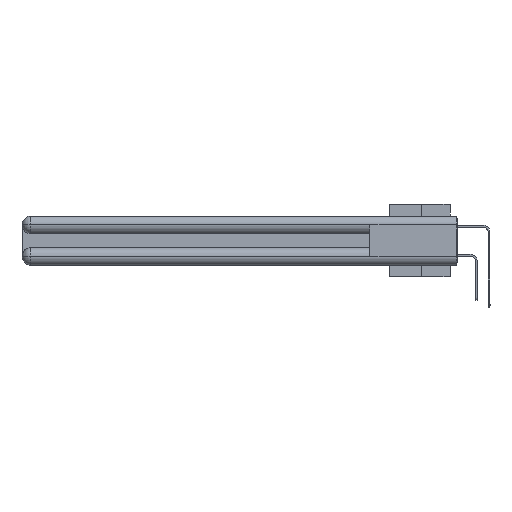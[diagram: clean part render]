
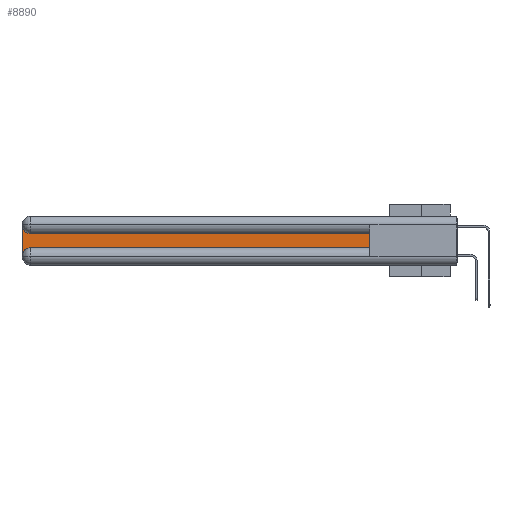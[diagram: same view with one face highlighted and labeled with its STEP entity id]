
A CAD part, left-side view. The second image highlights one B-rep face of the part: STEP entity #8890.
In plain terms, the highlighted planar face has unit normal (-1, 0, 0).
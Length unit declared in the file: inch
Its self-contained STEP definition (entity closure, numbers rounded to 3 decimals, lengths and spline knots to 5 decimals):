
#895 = DIRECTION ( 'NONE',  ( 0., 0., -1. ) ) ;
#2428 = DIRECTION ( 'NONE',  ( 0., 0., -1. ) ) ;
#3851 = CARTESIAN_POINT ( 'NONE',  ( 0.075, 2.94, -0.0625 ) ) ;
#4328 = EDGE_CURVE ( 'NONE', #30875, #16803, #29449, .T. ) ;
#4481 = VECTOR ( 'NONE', #14799, 39.37008 ) ;
#5250 = VERTEX_POINT ( 'NONE', #31226 ) ;
#7126 = DIRECTION ( 'NONE',  ( 1., 0., 0. ) ) ;
#7309 = PLANE ( 'NONE',  #14529 ) ;
#8488 = CARTESIAN_POINT ( 'NONE',  ( 0.075, 3., -0.2175 ) ) ;
#8618 = ORIENTED_EDGE ( 'NONE', *, *, #10377, .T. ) ;
#8878 = EDGE_CURVE ( 'NONE', #16803, #32591, #31275, .T. ) ;
#8890 = ADVANCED_FACE ( 'NONE', ( #12181 ), #7309, .F. ) ;
#8971 = DIRECTION ( 'NONE',  ( 1., 0., 0. ) ) ;
#9100 = CARTESIAN_POINT ( 'NONE',  ( 0.075, 3., -0.2775 ) ) ;
#10290 = CARTESIAN_POINT ( 'NONE',  ( 0.075, 2.94, -0.2175 ) ) ;
#10377 = EDGE_CURVE ( 'NONE', #29912, #5250, #31632, .T. ) ;
#10591 = CARTESIAN_POINT ( 'NONE',  ( 0.075, 2.94, -0.1225 ) ) ;
#10624 = CARTESIAN_POINT ( 'NONE',  ( 0.075, 0.6, -0.1225 ) ) ;
#11727 = ORIENTED_EDGE ( 'NONE', *, *, #4328, .T. ) ;
#11822 = CARTESIAN_POINT ( 'NONE',  ( 0.075, 0.6, -0.1225 ) ) ;
#12181 = FACE_OUTER_BOUND ( 'NONE', #33386, .T. ) ;
#12590 = CARTESIAN_POINT ( 'NONE',  ( 0.075, 0.6, -0.2175 ) ) ;
#12849 = ORIENTED_EDGE ( 'NONE', *, *, #33581, .T. ) ;
#13400 = CARTESIAN_POINT ( 'NONE',  ( 0.075, 2.94, -0.2775 ) ) ;
#13712 = AXIS2_PLACEMENT_3D ( 'NONE', #3851, #13789, #895 ) ;
#13789 = DIRECTION ( 'NONE',  ( 1., 0., 0. ) ) ;
#14529 = AXIS2_PLACEMENT_3D ( 'NONE', #22858, #7126, #23037 ) ;
#14799 = DIRECTION ( 'NONE',  ( 0., 0., 1. ) ) ;
#14837 = ORIENTED_EDGE ( 'NONE', *, *, #32232, .T. ) ;
#16380 = LINE ( 'NONE', #10624, #28019 ) ;
#16640 = DIRECTION ( 'NONE',  ( 0., -1., 0. ) ) ;
#16803 = VERTEX_POINT ( 'NONE', #12590 ) ;
#17849 = CIRCLE ( 'NONE', #30199, 0.06 ) ;
#21730 = EDGE_CURVE ( 'NONE', #5250, #29297, #24543, .T. ) ;
#22858 = CARTESIAN_POINT ( 'NONE',  ( 0.075, 3., -0.1225 ) ) ;
#23037 = DIRECTION ( 'NONE',  ( 0., 0., -1. ) ) ;
#23208 = CARTESIAN_POINT ( 'NONE',  ( 0.075, 0.6, -0.2175 ) ) ;
#24011 = CARTESIAN_POINT ( 'NONE',  ( 0.075, 0.6, -0.2175 ) ) ;
#24543 = LINE ( 'NONE', #8488, #26390 ) ;
#24870 = ORIENTED_EDGE ( 'NONE', *, *, #8878, .T. ) ;
#25335 = VECTOR ( 'NONE', #16640, 39.37008 ) ;
#26390 = VECTOR ( 'NONE', #29823, 39.37008 ) ;
#28019 = VECTOR ( 'NONE', #29524, 39.37008 ) ;
#28683 = ORIENTED_EDGE ( 'NONE', *, *, #21730, .T. ) ;
#29297 = VERTEX_POINT ( 'NONE', #9100 ) ;
#29449 = LINE ( 'NONE', #24011, #25335 ) ;
#29524 = DIRECTION ( 'NONE',  ( 0., 1., 0. ) ) ;
#29823 = DIRECTION ( 'NONE',  ( 0., 0., -1. ) ) ;
#29912 = VERTEX_POINT ( 'NONE', #10591 ) ;
#30199 = AXIS2_PLACEMENT_3D ( 'NONE', #13400, #8971, #2428 ) ;
#30875 = VERTEX_POINT ( 'NONE', #10290 ) ;
#31226 = CARTESIAN_POINT ( 'NONE',  ( 0.075, 3., -0.0625 ) ) ;
#31275 = LINE ( 'NONE', #23208, #4481 ) ;
#31632 = CIRCLE ( 'NONE', #13712, 0.06 ) ;
#32232 = EDGE_CURVE ( 'NONE', #29297, #30875, #17849, .T. ) ;
#32591 = VERTEX_POINT ( 'NONE', #11822 ) ;
#33386 = EDGE_LOOP ( 'NONE', ( #12849, #8618, #28683, #14837, #11727, #24870 ) ) ;
#33581 = EDGE_CURVE ( 'NONE', #32591, #29912, #16380, .T. ) ;
